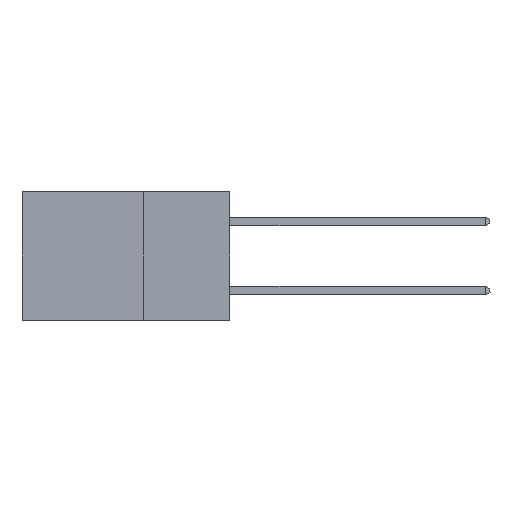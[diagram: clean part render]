
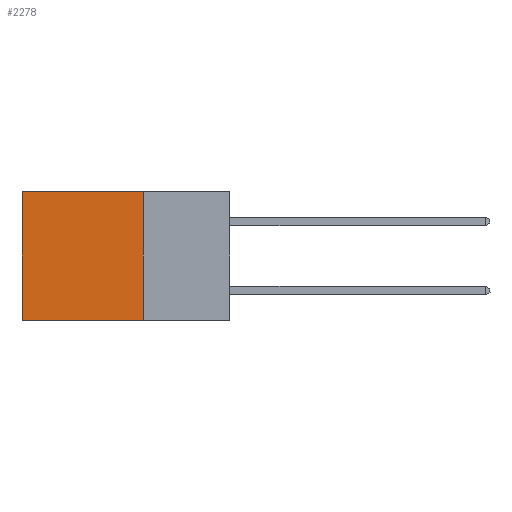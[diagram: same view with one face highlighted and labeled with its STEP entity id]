
A CAD part, left-side view. The second image highlights one B-rep face of the part: STEP entity #2278.
In plain terms, the highlighted planar face has unit normal (-1, 0, 0).
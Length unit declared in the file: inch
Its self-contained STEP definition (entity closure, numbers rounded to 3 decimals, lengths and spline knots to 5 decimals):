
#851 = CARTESIAN_POINT ( 'NONE',  ( 0.298, 0.25, 0. ) ) ;
#935 = ORIENTED_EDGE ( 'NONE', *, *, #2650, .F. ) ;
#1562 = DIRECTION ( 'NONE',  ( 0., 0., -1. ) ) ;
#1776 = DIRECTION ( 'NONE',  ( 0., 1., 0. ) ) ;
#2258 = VERTEX_POINT ( 'NONE', #4565 ) ;
#2278 = ADVANCED_FACE ( 'NONE', ( #13067 ), #17581, .F. ) ;
#2636 = LINE ( 'NONE', #851, #12831 ) ;
#2650 = EDGE_CURVE ( 'NONE', #19000, #2258, #8587, .T. ) ;
#2940 = EDGE_CURVE ( 'NONE', #3456, #16148, #13311, .T. ) ;
#3456 = VERTEX_POINT ( 'NONE', #11242 ) ;
#3752 = EDGE_CURVE ( 'NONE', #3456, #19000, #2636, .T. ) ;
#4565 = CARTESIAN_POINT ( 'NONE',  ( 0.298, 0.6, -0.37 ) ) ;
#4837 = CARTESIAN_POINT ( 'NONE',  ( 0.298, 0.25, -0.37 ) ) ;
#5303 = ORIENTED_EDGE ( 'NONE', *, *, #3752, .F. ) ;
#5952 = LINE ( 'NONE', #12322, #11184 ) ;
#6027 = DIRECTION ( 'NONE',  ( 0., 0., -1. ) ) ;
#6150 = CARTESIAN_POINT ( 'NONE',  ( 0.298, 0.25, 0. ) ) ;
#7943 = DIRECTION ( 'NONE',  ( 1., 0., 0. ) ) ;
#8587 = LINE ( 'NONE', #4837, #11327 ) ;
#8860 = CARTESIAN_POINT ( 'NONE',  ( 0.298, 0.6, 0. ) ) ;
#11184 = VECTOR ( 'NONE', #6027, 39.37008 ) ;
#11242 = CARTESIAN_POINT ( 'NONE',  ( 0.298, 0.25, 0. ) ) ;
#11327 = VECTOR ( 'NONE', #1776, 39.37008 ) ;
#12302 = DIRECTION ( 'NONE',  ( 0., 1., 0. ) ) ;
#12322 = CARTESIAN_POINT ( 'NONE',  ( 0.298, 0.6, 0. ) ) ;
#12545 = VECTOR ( 'NONE', #12302, 39.37008 ) ;
#12610 = CARTESIAN_POINT ( 'NONE',  ( 0.298, 0.25, 0. ) ) ;
#12630 = AXIS2_PLACEMENT_3D ( 'NONE', #12610, #7943, #1562 ) ;
#12831 = VECTOR ( 'NONE', #15339, 39.37008 ) ;
#13067 = FACE_OUTER_BOUND ( 'NONE', #15313, .T. ) ;
#13311 = LINE ( 'NONE', #6150, #12545 ) ;
#14815 = ORIENTED_EDGE ( 'NONE', *, *, #18336, .T. ) ;
#15313 = EDGE_LOOP ( 'NONE', ( #14815, #935, #5303, #18396 ) ) ;
#15339 = DIRECTION ( 'NONE',  ( 0., 0., -1. ) ) ;
#16148 = VERTEX_POINT ( 'NONE', #8860 ) ;
#16837 = CARTESIAN_POINT ( 'NONE',  ( 0.298, 0.25, -0.37 ) ) ;
#17581 = PLANE ( 'NONE',  #12630 ) ;
#18336 = EDGE_CURVE ( 'NONE', #16148, #2258, #5952, .T. ) ;
#18396 = ORIENTED_EDGE ( 'NONE', *, *, #2940, .T. ) ;
#19000 = VERTEX_POINT ( 'NONE', #16837 ) ;
